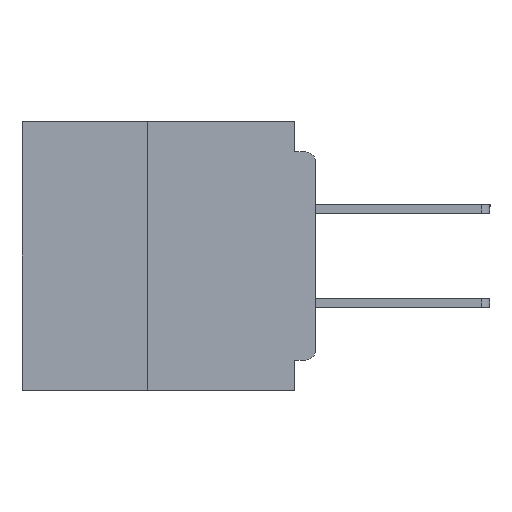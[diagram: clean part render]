
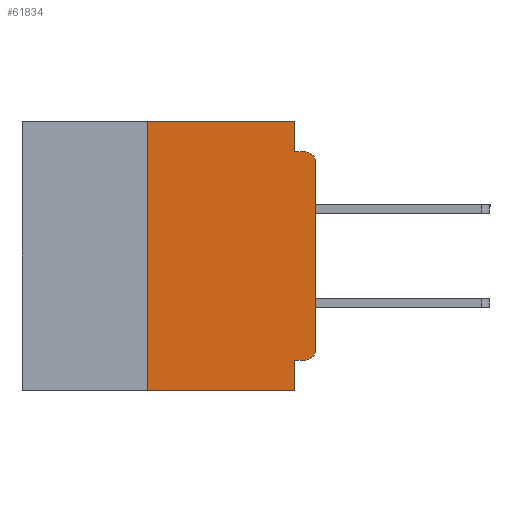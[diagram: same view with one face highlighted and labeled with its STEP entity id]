
A CAD part, left-side view. The second image highlights one B-rep face of the part: STEP entity #61834.
In plain terms, the highlighted planar face has unit normal (-1, 0, 0).
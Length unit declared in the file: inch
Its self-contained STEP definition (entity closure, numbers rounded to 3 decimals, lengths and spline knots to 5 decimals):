
#2990 = LINE ( 'NONE', #11193, #40183 ) ;
#3975 = CARTESIAN_POINT ( 'NONE',  ( 0., 0., 0. ) ) ;
#4392 = CARTESIAN_POINT ( 'NONE',  ( 0., 0., -0.045 ) ) ;
#8849 = DIRECTION ( 'NONE',  ( 0., 0., 1. ) ) ;
#9230 = DIRECTION ( 'NONE',  ( 0., -1., 0. ) ) ;
#10397 = VERTEX_POINT ( 'NONE', #10982 ) ;
#10982 = CARTESIAN_POINT ( 'NONE',  ( 0., 0.031, -0.4 ) ) ;
#11193 = CARTESIAN_POINT ( 'NONE',  ( 0., 0.031, -0.4 ) ) ;
#11909 = EDGE_CURVE ( 'NONE', #26537, #17638, #16297, .T. ) ;
#13327 = LINE ( 'NONE', #18595, #53528 ) ;
#15321 = EDGE_CURVE ( 'NONE', #17638, #44135, #41762, .T. ) ;
#15790 = ORIENTED_EDGE ( 'NONE', *, *, #52962, .F. ) ;
#16073 = DIRECTION ( 'NONE',  ( 0., 0., -1. ) ) ;
#16297 = CIRCLE ( 'NONE', #29209, 0.015 ) ;
#17366 = DIRECTION ( 'NONE',  ( 0., -1., 0. ) ) ;
#17638 = VERTEX_POINT ( 'NONE', #45933 ) ;
#17997 = CARTESIAN_POINT ( 'NONE',  ( 0., 0.015, -0.34 ) ) ;
#18595 = CARTESIAN_POINT ( 'NONE',  ( 0., 0.437, -0.4 ) ) ;
#20409 = EDGE_CURVE ( 'NONE', #44135, #61100, #41344, .T. ) ;
#20424 = CARTESIAN_POINT ( 'NONE',  ( 0., 0.015, -0.06 ) ) ;
#22617 = PLANE ( 'NONE',  #39235 ) ;
#22752 = LINE ( 'NONE', #57566, #59865 ) ;
#22828 = DIRECTION ( 'NONE',  ( 1., 0., 0. ) ) ;
#22871 = DIRECTION ( 'NONE',  ( 0., 0., -1. ) ) ;
#23484 = CARTESIAN_POINT ( 'NONE',  ( 0., 0.25, -0.4 ) ) ;
#23700 = VECTOR ( 'NONE', #9230, 39.37008 ) ;
#25310 = DIRECTION ( 'NONE',  ( 0., 0., -1. ) ) ;
#26293 = CARTESIAN_POINT ( 'NONE',  ( 0., 0.031, 0. ) ) ;
#26305 = CARTESIAN_POINT ( 'NONE',  ( 0., 0.015, -0.045 ) ) ;
#26537 = VERTEX_POINT ( 'NONE', #36574 ) ;
#27915 = ORIENTED_EDGE ( 'NONE', *, *, #31060, .F. ) ;
#28617 = EDGE_CURVE ( 'NONE', #29653, #61100, #42713, .T. ) ;
#28864 = CARTESIAN_POINT ( 'NONE',  ( 0., 0.25, 0. ) ) ;
#29209 = AXIS2_PLACEMENT_3D ( 'NONE', #17997, #51922, #22871 ) ;
#29653 = VERTEX_POINT ( 'NONE', #55498 ) ;
#31060 = EDGE_CURVE ( 'NONE', #34682, #49430, #56154, .T. ) ;
#32302 = EDGE_CURVE ( 'NONE', #26537, #40288, #22752, .T. ) ;
#32945 = CARTESIAN_POINT ( 'NONE',  ( 0., 0.25, -0.4 ) ) ;
#33519 = VECTOR ( 'NONE', #47438, 39.37008 ) ;
#34682 = VERTEX_POINT ( 'NONE', #23484 ) ;
#36574 = CARTESIAN_POINT ( 'NONE',  ( 0., 0.015, -0.355 ) ) ;
#36588 = ORIENTED_EDGE ( 'NONE', *, *, #53121, .T. ) ;
#39235 = AXIS2_PLACEMENT_3D ( 'NONE', #51880, #22828, #56694 ) ;
#40183 = VECTOR ( 'NONE', #16073, 39.37008 ) ;
#40288 = VERTEX_POINT ( 'NONE', #54076 ) ;
#40771 = ORIENTED_EDGE ( 'NONE', *, *, #11909, .T. ) ;
#41344 = CIRCLE ( 'NONE', #50853, 0.015 ) ;
#41762 = LINE ( 'NONE', #3975, #51589 ) ;
#41802 = VECTOR ( 'NONE', #52037, 39.37008 ) ;
#42560 = CARTESIAN_POINT ( 'NONE',  ( 0., 0.031, 0. ) ) ;
#42653 = EDGE_CURVE ( 'NONE', #52887, #29653, #59266, .T. ) ;
#42713 = LINE ( 'NONE', #4392, #23700 ) ;
#44135 = VERTEX_POINT ( 'NONE', #54204 ) ;
#45933 = CARTESIAN_POINT ( 'NONE',  ( 0., 0., -0.34 ) ) ;
#47438 = DIRECTION ( 'NONE',  ( 0., 0., -1. ) ) ;
#47694 = DIRECTION ( 'NONE',  ( 0., -1., 0. ) ) ;
#48278 = LINE ( 'NONE', #60735, #59571 ) ;
#49430 = VERTEX_POINT ( 'NONE', #28864 ) ;
#50853 = AXIS2_PLACEMENT_3D ( 'NONE', #20424, #54338, #25310 ) ;
#51589 = VECTOR ( 'NONE', #8849, 39.37008 ) ;
#51880 = CARTESIAN_POINT ( 'NONE',  ( 0., 0.437, 0. ) ) ;
#51922 = DIRECTION ( 'NONE',  ( -1., 0., 0. ) ) ;
#52037 = DIRECTION ( 'NONE',  ( 0., 0., 1. ) ) ;
#52712 = ORIENTED_EDGE ( 'NONE', *, *, #32302, .F. ) ;
#52887 = VERTEX_POINT ( 'NONE', #26293 ) ;
#52962 = EDGE_CURVE ( 'NONE', #49430, #52887, #48278, .T. ) ;
#53121 = EDGE_CURVE ( 'NONE', #34682, #10397, #13327, .T. ) ;
#53528 = VECTOR ( 'NONE', #47694, 39.37008 ) ;
#54076 = CARTESIAN_POINT ( 'NONE',  ( 0., 0.031, -0.355 ) ) ;
#54204 = CARTESIAN_POINT ( 'NONE',  ( 0., 0., -0.06 ) ) ;
#54338 = DIRECTION ( 'NONE',  ( -1., 0., 0. ) ) ;
#55498 = CARTESIAN_POINT ( 'NONE',  ( 0., 0.031, -0.045 ) ) ;
#55612 = ORIENTED_EDGE ( 'NONE', *, *, #42653, .F. ) ;
#56154 = LINE ( 'NONE', #32945, #41802 ) ;
#56694 = DIRECTION ( 'NONE',  ( 0., 0., -1. ) ) ;
#57370 = EDGE_LOOP ( 'NONE', ( #62635, #61598, #60506, #55612, #15790, #27915, #36588, #61550, #52712, #40771 ) ) ;
#57566 = CARTESIAN_POINT ( 'NONE',  ( 0., 0., -0.355 ) ) ;
#58807 = FACE_OUTER_BOUND ( 'NONE', #57370, .T. ) ;
#59266 = LINE ( 'NONE', #42560, #33519 ) ;
#59571 = VECTOR ( 'NONE', #17366, 39.37008 ) ;
#59747 = EDGE_CURVE ( 'NONE', #40288, #10397, #2990, .T. ) ;
#59865 = VECTOR ( 'NONE', #62425, 39.37008 ) ;
#60506 = ORIENTED_EDGE ( 'NONE', *, *, #28617, .F. ) ;
#60735 = CARTESIAN_POINT ( 'NONE',  ( 0., 0.437, 0. ) ) ;
#61100 = VERTEX_POINT ( 'NONE', #26305 ) ;
#61550 = ORIENTED_EDGE ( 'NONE', *, *, #59747, .F. ) ;
#61598 = ORIENTED_EDGE ( 'NONE', *, *, #20409, .T. ) ;
#61834 = ADVANCED_FACE ( 'NONE', ( #58807 ), #22617, .F. ) ;
#62425 = DIRECTION ( 'NONE',  ( 0., 1., 0. ) ) ;
#62635 = ORIENTED_EDGE ( 'NONE', *, *, #15321, .T. ) ;
